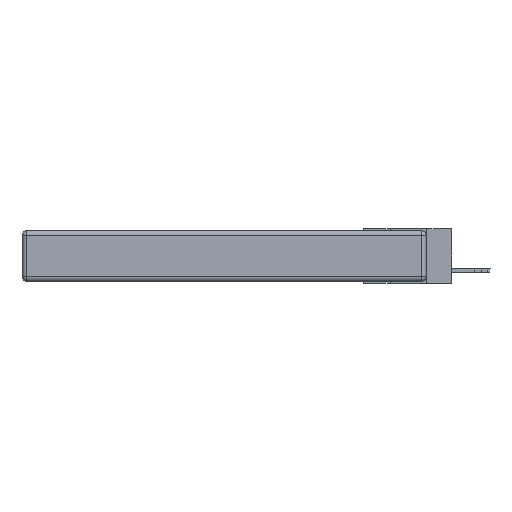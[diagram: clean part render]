
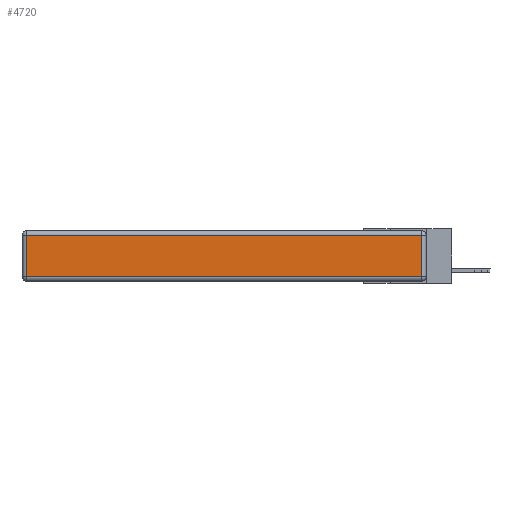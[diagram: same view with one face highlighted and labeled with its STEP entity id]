
A CAD part, left-side view. The second image highlights one B-rep face of the part: STEP entity #4720.
In plain terms, the highlighted planar face has unit normal (-1, 0, 0).
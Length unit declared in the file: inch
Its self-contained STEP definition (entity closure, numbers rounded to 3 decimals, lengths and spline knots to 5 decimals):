
#82 = DIRECTION ( 'NONE',  ( -1., 0., 0. ) ) ;
#949 = EDGE_LOOP ( 'NONE', ( #4551, #11205, #11602, #10609 ) ) ;
#1033 = VECTOR ( 'NONE', #3922, 39.37008 ) ;
#1268 = CARTESIAN_POINT ( 'NONE',  ( 0., 2.72, -0.313 ) ) ;
#1425 = VERTEX_POINT ( 'NONE', #1268 ) ;
#1512 = FACE_OUTER_BOUND ( 'NONE', #949, .T. ) ;
#1848 = LINE ( 'NONE', #12055, #8593 ) ;
#2649 = DIRECTION ( 'NONE',  ( 0., 0., 1. ) ) ;
#2734 = CARTESIAN_POINT ( 'NONE',  ( 0., 2.72, -0.03 ) ) ;
#3391 = DIRECTION ( 'NONE',  ( 0., 0., 1. ) ) ;
#3922 = DIRECTION ( 'NONE',  ( 0., 1., 0. ) ) ;
#4551 = ORIENTED_EDGE ( 'NONE', *, *, #5073, .T. ) ;
#4720 = ADVANCED_FACE ( 'NONE', ( #1512 ), #5613, .T. ) ;
#5073 = EDGE_CURVE ( 'NONE', #1425, #13148, #1848, .T. ) ;
#5613 = PLANE ( 'NONE',  #10932 ) ;
#5809 = CARTESIAN_POINT ( 'NONE',  ( 0., 0.03, -0.343 ) ) ;
#6730 = CARTESIAN_POINT ( 'NONE',  ( 0., 0., -0.343 ) ) ;
#7367 = DIRECTION ( 'NONE',  ( 0., 0., -1. ) ) ;
#7390 = CARTESIAN_POINT ( 'NONE',  ( 0., 2.75, -0.03 ) ) ;
#7610 = DIRECTION ( 'NONE',  ( 0., -1., 0. ) ) ;
#7917 = VECTOR ( 'NONE', #7367, 39.37008 ) ;
#8593 = VECTOR ( 'NONE', #7610, 39.37008 ) ;
#8648 = LINE ( 'NONE', #7390, #1033 ) ;
#10478 = LINE ( 'NONE', #5809, #12961 ) ;
#10589 = EDGE_CURVE ( 'NONE', #12413, #1425, #13735, .T. ) ;
#10609 = ORIENTED_EDGE ( 'NONE', *, *, #10589, .T. ) ;
#10858 = CARTESIAN_POINT ( 'NONE',  ( 0., 0.03, -0.03 ) ) ;
#10932 = AXIS2_PLACEMENT_3D ( 'NONE', #6730, #82, #3391 ) ;
#11205 = ORIENTED_EDGE ( 'NONE', *, *, #13137, .T. ) ;
#11394 = EDGE_CURVE ( 'NONE', #12657, #12413, #8648, .T. ) ;
#11602 = ORIENTED_EDGE ( 'NONE', *, *, #11394, .T. ) ;
#12055 = CARTESIAN_POINT ( 'NONE',  ( 0., 0., -0.313 ) ) ;
#12413 = VERTEX_POINT ( 'NONE', #2734 ) ;
#12640 = CARTESIAN_POINT ( 'NONE',  ( 0., 0.03, -0.313 ) ) ;
#12657 = VERTEX_POINT ( 'NONE', #10858 ) ;
#12961 = VECTOR ( 'NONE', #2649, 39.37008 ) ;
#13137 = EDGE_CURVE ( 'NONE', #13148, #12657, #10478, .T. ) ;
#13148 = VERTEX_POINT ( 'NONE', #12640 ) ;
#13735 = LINE ( 'NONE', #14028, #7917 ) ;
#14028 = CARTESIAN_POINT ( 'NONE',  ( 0., 2.72, -0.343 ) ) ;
